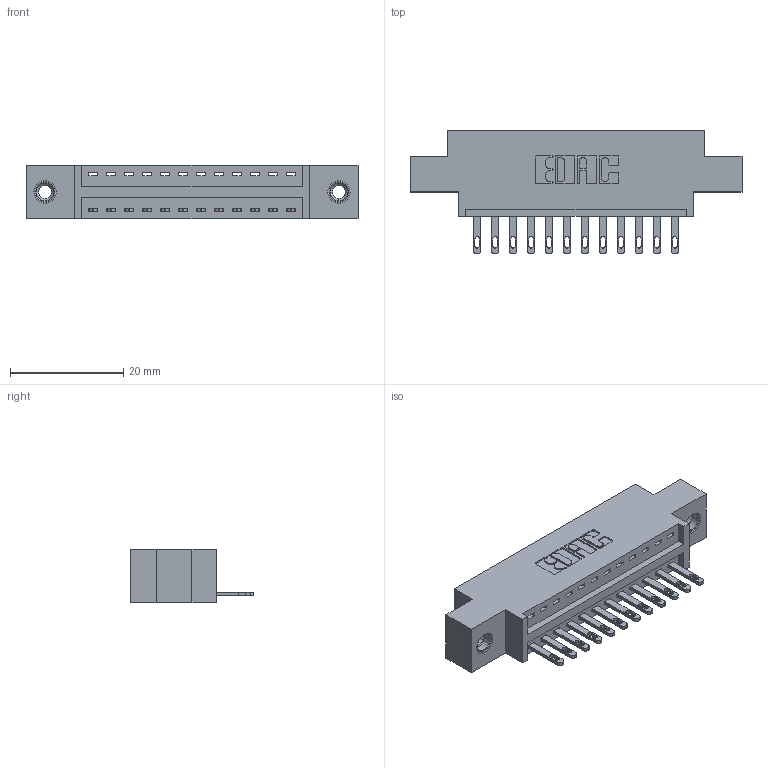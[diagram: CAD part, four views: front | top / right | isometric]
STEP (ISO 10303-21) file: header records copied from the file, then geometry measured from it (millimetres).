
FILE_DESCRIPTION (( 'STEP AP203' ), '1' );
FILE_NAME ('896-012-500-608.STEP', '2021-07-27T14:51:54', ( '' ), ( '' ), 'SwSTEP 2.0', 'SolidWorks 2020', '' );
FILE_SCHEMA (( 'CONFIG_CONTROL_DESIGN' ));
Length unit declared in the file: inch
Products named in the file (4): 345-250-001_345-250-003-102; 345-292-001_345-293-100; 896-012-500-608; 846 Part_0.170 Offset - 0.156 Dia-TI
Assembly tree (15 placements, depth 2):
  896-012-500-608
    846 Part_0.170 Offset - 0.156 Dia-TI
    345-292-001_345-293-100  x12
    345-250-001_345-250-003-102  x2
Bounding box: 58.67 x 21.84 x 9.4 mm (x, y, z)
Volume: 5256 mm3; surface area: 6455.7 mm2
Topology: 15 solids, 15 shells, 834 faces, 2493 edges, 1654 vertices
Faces by surface type: plane 520, cylinder 298, cone 12, torus 4
Entity records: 12734 total; most frequent: CARTESIAN_POINT 2175, ORIENTED_EDGE 2114, DIRECTION 1983, EDGE_CURVE 1057, LINE 853, VECTOR 853, VERTEX_POINT 700, AXIS2_PLACEMENT_3D 565
